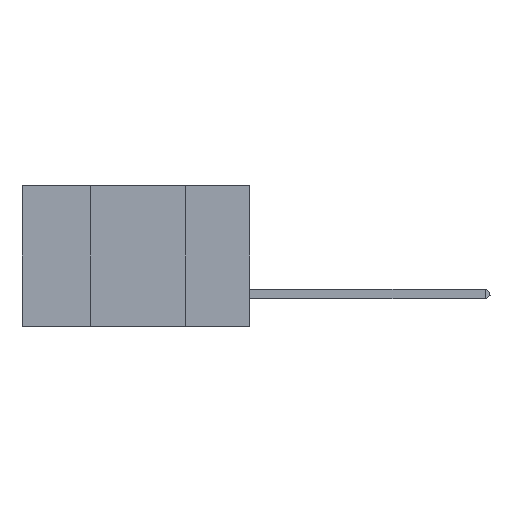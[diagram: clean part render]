
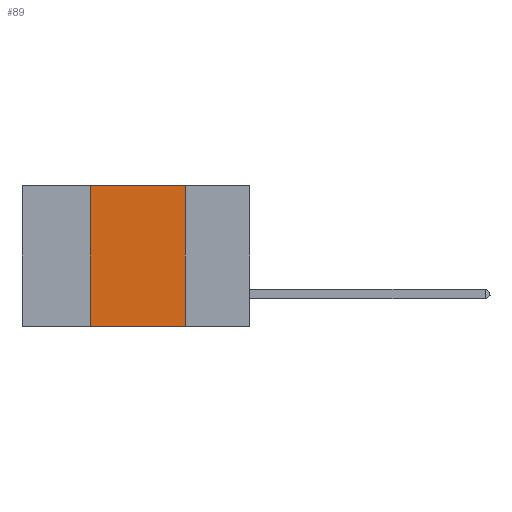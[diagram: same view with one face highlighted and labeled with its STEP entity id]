
A CAD part, left-side view. The second image highlights one B-rep face of the part: STEP entity #89.
In plain terms, the highlighted planar face has unit normal (-1, 0, 0).
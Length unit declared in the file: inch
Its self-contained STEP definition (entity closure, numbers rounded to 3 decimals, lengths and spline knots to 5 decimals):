
#82 = VECTOR ( 'NONE', #23383, 39.37008 ) ;
#89 = ADVANCED_FACE ( 'NONE', ( #19283 ), #17127, .F. ) ;
#352 = VECTOR ( 'NONE', #27317, 39.37008 ) ;
#2436 = AXIS2_PLACEMENT_3D ( 'NONE', #21288, #8053, #21606 ) ;
#3488 = EDGE_CURVE ( 'NONE', #16038, #10208, #27960, .T. ) ;
#3762 = VECTOR ( 'NONE', #4877, 39.37008 ) ;
#4877 = DIRECTION ( 'NONE',  ( 0., -1., 0. ) ) ;
#5574 = CARTESIAN_POINT ( 'NONE',  ( 0., 0.42, 0. ) ) ;
#7456 = EDGE_CURVE ( 'NONE', #24778, #10208, #14231, .T. ) ;
#7717 = EDGE_LOOP ( 'NONE', ( #18599, #21189, #12389, #9127 ) ) ;
#8053 = DIRECTION ( 'NONE',  ( 1., 0., 0. ) ) ;
#9127 = ORIENTED_EDGE ( 'NONE', *, *, #3488, .T. ) ;
#9148 = CARTESIAN_POINT ( 'NONE',  ( 0., 0.6, -0.37 ) ) ;
#9380 = EDGE_CURVE ( 'NONE', #16038, #11766, #17728, .T. ) ;
#10208 = VERTEX_POINT ( 'NONE', #10431 ) ;
#10431 = CARTESIAN_POINT ( 'NONE',  ( 0., 0.17, -0.37 ) ) ;
#11537 = EDGE_CURVE ( 'NONE', #11766, #24778, #18633, .T. ) ;
#11741 = CARTESIAN_POINT ( 'NONE',  ( 0., 0.17, 0. ) ) ;
#11766 = VERTEX_POINT ( 'NONE', #5574 ) ;
#12389 = ORIENTED_EDGE ( 'NONE', *, *, #9380, .F. ) ;
#13566 = CARTESIAN_POINT ( 'NONE',  ( 0., 0.42, 0. ) ) ;
#14074 = CARTESIAN_POINT ( 'NONE',  ( 0., 0.6, 0. ) ) ;
#14231 = LINE ( 'NONE', #27520, #82 ) ;
#14515 = CARTESIAN_POINT ( 'NONE',  ( 0., 0.42, -0.37 ) ) ;
#16038 = VERTEX_POINT ( 'NONE', #14515 ) ;
#16247 = DIRECTION ( 'NONE',  ( 0., -1., 0. ) ) ;
#17127 = PLANE ( 'NONE',  #2436 ) ;
#17728 = LINE ( 'NONE', #13566, #352 ) ;
#18599 = ORIENTED_EDGE ( 'NONE', *, *, #7456, .F. ) ;
#18633 = LINE ( 'NONE', #14074, #3762 ) ;
#19283 = FACE_OUTER_BOUND ( 'NONE', #7717, .T. ) ;
#21189 = ORIENTED_EDGE ( 'NONE', *, *, #11537, .F. ) ;
#21288 = CARTESIAN_POINT ( 'NONE',  ( 0., 0.6, 0. ) ) ;
#21606 = DIRECTION ( 'NONE',  ( 0., 0., -1. ) ) ;
#21977 = VECTOR ( 'NONE', #16247, 39.37008 ) ;
#23383 = DIRECTION ( 'NONE',  ( 0., 0., -1. ) ) ;
#24778 = VERTEX_POINT ( 'NONE', #11741 ) ;
#27317 = DIRECTION ( 'NONE',  ( 0., 0., 1. ) ) ;
#27520 = CARTESIAN_POINT ( 'NONE',  ( 0., 0.17, 0. ) ) ;
#27960 = LINE ( 'NONE', #9148, #21977 ) ;
